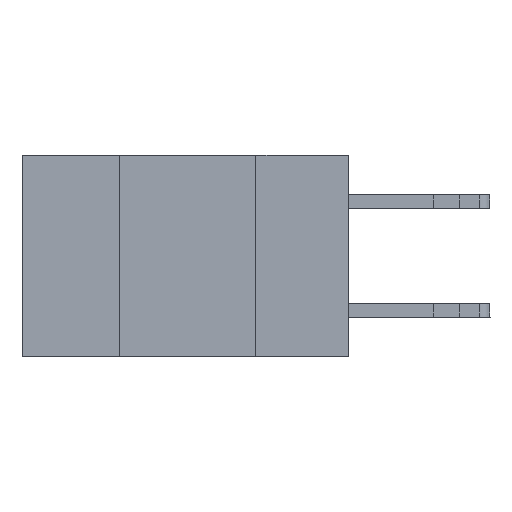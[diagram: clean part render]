
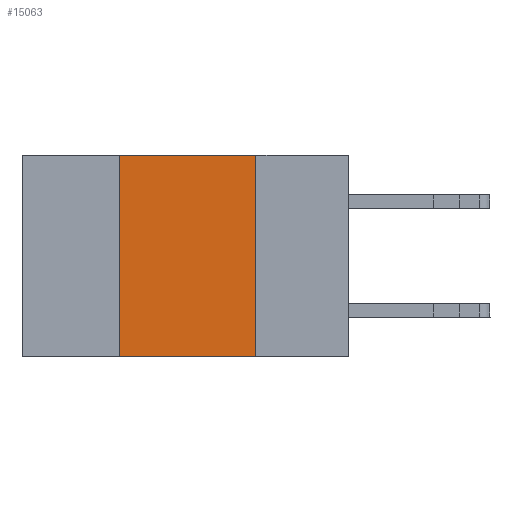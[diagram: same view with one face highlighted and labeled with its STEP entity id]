
A CAD part, left-side view. The second image highlights one B-rep face of the part: STEP entity #15063.
In plain terms, the highlighted planar face has unit normal (-1, 0, 0).
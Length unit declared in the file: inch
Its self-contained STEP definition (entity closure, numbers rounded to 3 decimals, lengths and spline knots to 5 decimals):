
#158 = VERTEX_POINT ( 'NONE', #3160 ) ;
#178 = ORIENTED_EDGE ( 'NONE', *, *, #20285, .F. ) ;
#676 = VERTEX_POINT ( 'NONE', #6308 ) ;
#863 = VECTOR ( 'NONE', #18497, 39.37008 ) ;
#1109 = ORIENTED_EDGE ( 'NONE', *, *, #8221, .F. ) ;
#1727 = VERTEX_POINT ( 'NONE', #5408 ) ;
#2930 = LINE ( 'NONE', #9036, #15387 ) ;
#3160 = CARTESIAN_POINT ( 'NONE',  ( 0., 0.42, 0. ) ) ;
#4817 = CARTESIAN_POINT ( 'NONE',  ( 0., 0.17, -0.37 ) ) ;
#5408 = CARTESIAN_POINT ( 'NONE',  ( 0., 0.17, 0. ) ) ;
#6308 = CARTESIAN_POINT ( 'NONE',  ( 0., 0.42, -0.37 ) ) ;
#6325 = CARTESIAN_POINT ( 'NONE',  ( 0., 0.6, -0.37 ) ) ;
#7385 = DIRECTION ( 'NONE',  ( 0., 0., -1. ) ) ;
#7731 = EDGE_LOOP ( 'NONE', ( #178, #1109, #14173, #8188 ) ) ;
#7760 = LINE ( 'NONE', #17710, #20178 ) ;
#8026 = EDGE_CURVE ( 'NONE', #676, #158, #2930, .T. ) ;
#8188 = ORIENTED_EDGE ( 'NONE', *, *, #20016, .T. ) ;
#8221 = EDGE_CURVE ( 'NONE', #158, #1727, #7760, .T. ) ;
#9036 = CARTESIAN_POINT ( 'NONE',  ( 0., 0.42, 0. ) ) ;
#9781 = LINE ( 'NONE', #6325, #16875 ) ;
#10402 = FACE_OUTER_BOUND ( 'NONE', #7731, .T. ) ;
#12884 = DIRECTION ( 'NONE',  ( 0., -1., 0. ) ) ;
#13256 = AXIS2_PLACEMENT_3D ( 'NONE', #17104, #17034, #7385 ) ;
#13317 = LINE ( 'NONE', #18564, #863 ) ;
#14173 = ORIENTED_EDGE ( 'NONE', *, *, #8026, .F. ) ;
#15063 = ADVANCED_FACE ( 'NONE', ( #10402 ), #20275, .F. ) ;
#15387 = VECTOR ( 'NONE', #15576, 39.37008 ) ;
#15576 = DIRECTION ( 'NONE',  ( 0., 0., 1. ) ) ;
#16334 = DIRECTION ( 'NONE',  ( 0., -1., 0. ) ) ;
#16820 = VERTEX_POINT ( 'NONE', #4817 ) ;
#16875 = VECTOR ( 'NONE', #16334, 39.37008 ) ;
#17034 = DIRECTION ( 'NONE',  ( 1., 0., 0. ) ) ;
#17104 = CARTESIAN_POINT ( 'NONE',  ( 0., 0.6, 0. ) ) ;
#17710 = CARTESIAN_POINT ( 'NONE',  ( 0., 0.6, 0. ) ) ;
#18497 = DIRECTION ( 'NONE',  ( 0., 0., -1. ) ) ;
#18564 = CARTESIAN_POINT ( 'NONE',  ( 0., 0.17, 0. ) ) ;
#20016 = EDGE_CURVE ( 'NONE', #676, #16820, #9781, .T. ) ;
#20178 = VECTOR ( 'NONE', #12884, 39.37008 ) ;
#20275 = PLANE ( 'NONE',  #13256 ) ;
#20285 = EDGE_CURVE ( 'NONE', #1727, #16820, #13317, .T. ) ;
